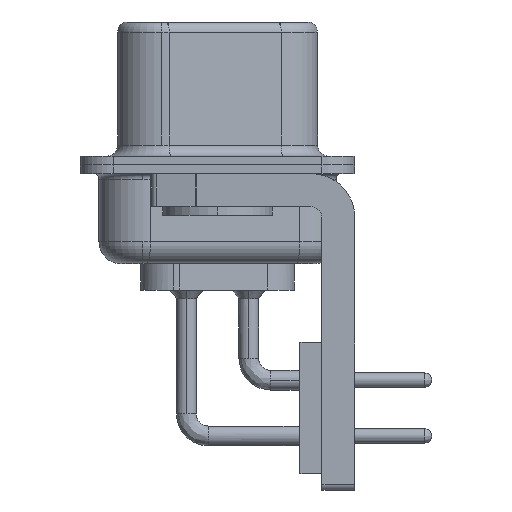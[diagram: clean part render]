
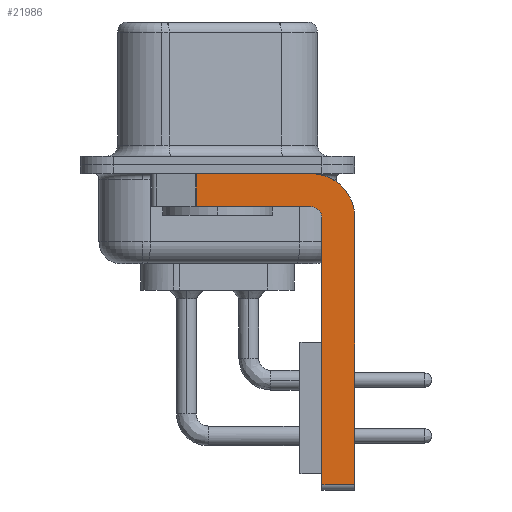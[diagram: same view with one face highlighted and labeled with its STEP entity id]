
A CAD part, left-side view. The second image highlights one B-rep face of the part: STEP entity #21986.
In plain terms, the highlighted planar face has unit normal (-1, 0, 0).
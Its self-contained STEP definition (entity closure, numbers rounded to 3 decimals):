
#790 = CARTESIAN_POINT ( 'NONE',  ( -2.9, -4.25, -14.55 ) ) ;
#1809 = VERTEX_POINT ( 'NONE', #29274 ) ;
#2348 = LINE ( 'NONE', #30232, #14992 ) ;
#2352 = VERTEX_POINT ( 'NONE', #25065 ) ;
#2817 = ORIENTED_EDGE ( 'NONE', *, *, #20010, .F. ) ;
#3014 = CARTESIAN_POINT ( 'NONE',  ( -2.9, -6.25, -2.4 ) ) ;
#3119 = DIRECTION ( 'NONE',  ( 0., 0., -1. ) ) ;
#3263 = CARTESIAN_POINT ( 'NONE',  ( -2.9, 0.978, -1.9 ) ) ;
#3395 = CARTESIAN_POINT ( 'NONE',  ( -2.9, -4.75, -14.55 ) ) ;
#3558 = DIRECTION ( 'NONE',  ( 0., -1., 0. ) ) ;
#6148 = EDGE_CURVE ( 'NONE', #16750, #15044, #2348, .T. ) ;
#6201 = VERTEX_POINT ( 'NONE', #29008 ) ;
#6211 = VERTEX_POINT ( 'NONE', #28586 ) ;
#6518 = CARTESIAN_POINT ( 'NONE',  ( -2.9, -4.25, -1.9 ) ) ;
#6585 = EDGE_CURVE ( 'NONE', #31606, #2352, #18320, .T. ) ;
#6613 = PLANE ( 'NONE',  #22707 ) ;
#6729 = DIRECTION ( 'NONE',  ( 0., 0., -1. ) ) ;
#7829 = AXIS2_PLACEMENT_3D ( 'NONE', #15415, #33552, #18131 ) ;
#7876 = AXIS2_PLACEMENT_3D ( 'NONE', #14484, #32687, #17199 ) ;
#8095 = EDGE_CURVE ( 'NONE', #6211, #6201, #10217, .T. ) ;
#9680 = EDGE_CURVE ( 'NONE', #15044, #17186, #20447, .T. ) ;
#10217 = LINE ( 'NONE', #3263, #31206 ) ;
#13038 = EDGE_CURVE ( 'NONE', #6211, #1809, #13170, .T. ) ;
#13170 = LINE ( 'NONE', #19628, #33138 ) ;
#14484 = CARTESIAN_POINT ( 'NONE',  ( -2.9, -4.25, -2.4 ) ) ;
#14556 = VECTOR ( 'NONE', #25158, 1000. ) ;
#14623 = ORIENTED_EDGE ( 'NONE', *, *, #9680, .F. ) ;
#14831 = CARTESIAN_POINT ( 'NONE',  ( -2.9, -4.75, -2.4 ) ) ;
#14992 = VECTOR ( 'NONE', #30115, 1000. ) ;
#15044 = VERTEX_POINT ( 'NONE', #14831 ) ;
#15090 = DIRECTION ( 'NONE',  ( 0., 0., -1. ) ) ;
#15415 = CARTESIAN_POINT ( 'NONE',  ( -2.9, -4.25, -2.4 ) ) ;
#16750 = VERTEX_POINT ( 'NONE', #3395 ) ;
#17186 = VERTEX_POINT ( 'NONE', #28963 ) ;
#17199 = DIRECTION ( 'NONE',  ( 0., 0., 1. ) ) ;
#17792 = FACE_OUTER_BOUND ( 'NONE', #24393, .T. ) ;
#18131 = DIRECTION ( 'NONE',  ( 0., 0., -1. ) ) ;
#18320 = LINE ( 'NONE', #3014, #24469 ) ;
#19054 = ORIENTED_EDGE ( 'NONE', *, *, #6585, .F. ) ;
#19628 = CARTESIAN_POINT ( 'NONE',  ( -2.9, 3., -0.4 ) ) ;
#20010 = EDGE_CURVE ( 'NONE', #17186, #6201, #33640, .T. ) ;
#20017 = ORIENTED_EDGE ( 'NONE', *, *, #25789, .F. ) ;
#20447 = CIRCLE ( 'NONE', #7876, 0.5 ) ;
#21986 = ADVANCED_FACE ( 'NONE', ( #17792 ), #6613, .F. ) ;
#22485 = EDGE_CURVE ( 'NONE', #16750, #2352, #32324, .T. ) ;
#22707 = AXIS2_PLACEMENT_3D ( 'NONE', #25240, #22736, #6729 ) ;
#22736 = DIRECTION ( 'NONE',  ( 1., 0., 0. ) ) ;
#24393 = EDGE_LOOP ( 'NONE', ( #31365, #26632, #2817, #14623, #30341, #29306, #19054, #20017 ) ) ;
#24469 = VECTOR ( 'NONE', #3119, 1000. ) ;
#24863 = DIRECTION ( 'NONE',  ( 0., -1., 0. ) ) ;
#25065 = CARTESIAN_POINT ( 'NONE',  ( -2.9, -6.25, -14.55 ) ) ;
#25158 = DIRECTION ( 'NONE',  ( 0., 1., 0. ) ) ;
#25240 = CARTESIAN_POINT ( 'NONE',  ( -2.9, -4.25, -2.4 ) ) ;
#25320 = CARTESIAN_POINT ( 'NONE',  ( -2.9, -6.25, -2.4 ) ) ;
#25789 = EDGE_CURVE ( 'NONE', #1809, #31606, #26088, .T. ) ;
#26088 = CIRCLE ( 'NONE', #7829, 2. ) ;
#26632 = ORIENTED_EDGE ( 'NONE', *, *, #8095, .T. ) ;
#28586 = CARTESIAN_POINT ( 'NONE',  ( -2.9, 0.978, -0.4 ) ) ;
#28963 = CARTESIAN_POINT ( 'NONE',  ( -2.9, -4.25, -1.9 ) ) ;
#29008 = CARTESIAN_POINT ( 'NONE',  ( -2.9, 0.978, -1.9 ) ) ;
#29274 = CARTESIAN_POINT ( 'NONE',  ( -2.9, -4.25, -0.4 ) ) ;
#29306 = ORIENTED_EDGE ( 'NONE', *, *, #22485, .T. ) ;
#30115 = DIRECTION ( 'NONE',  ( 0., 0., 1. ) ) ;
#30232 = CARTESIAN_POINT ( 'NONE',  ( -2.9, -4.75, -14.8 ) ) ;
#30341 = ORIENTED_EDGE ( 'NONE', *, *, #6148, .F. ) ;
#31206 = VECTOR ( 'NONE', #15090, 1000. ) ;
#31365 = ORIENTED_EDGE ( 'NONE', *, *, #13038, .F. ) ;
#31532 = VECTOR ( 'NONE', #24863, 1000. ) ;
#31606 = VERTEX_POINT ( 'NONE', #25320 ) ;
#32324 = LINE ( 'NONE', #790, #31532 ) ;
#32687 = DIRECTION ( 'NONE',  ( -1., 0., 0. ) ) ;
#33138 = VECTOR ( 'NONE', #3558, 1000. ) ;
#33552 = DIRECTION ( 'NONE',  ( 1., 0., 0. ) ) ;
#33640 = LINE ( 'NONE', #6518, #14556 ) ;
